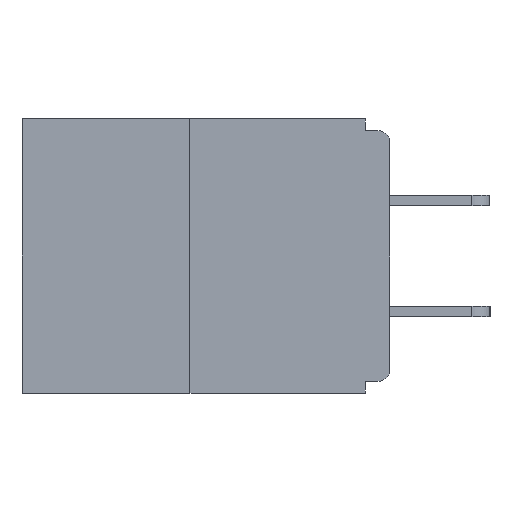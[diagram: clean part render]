
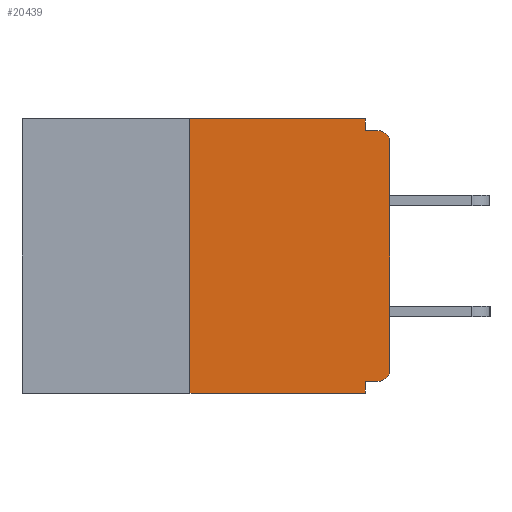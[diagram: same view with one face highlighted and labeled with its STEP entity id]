
A CAD part, left-side view. The second image highlights one B-rep face of the part: STEP entity #20439.
In plain terms, the highlighted planar face has unit normal (-1, 0, 0).
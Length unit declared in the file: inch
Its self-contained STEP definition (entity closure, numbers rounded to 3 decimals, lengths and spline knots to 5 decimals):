
#241 = CARTESIAN_POINT ( 'NONE',  ( 0., 0.015, -0.328 ) ) ;
#508 = CARTESIAN_POINT ( 'NONE',  ( 0., 0.031, -0.343 ) ) ;
#627 = LINE ( 'NONE', #2416, #22317 ) ;
#1248 = CARTESIAN_POINT ( 'NONE',  ( 0., 0., -0.03 ) ) ;
#1340 = VERTEX_POINT ( 'NONE', #13011 ) ;
#1684 = CARTESIAN_POINT ( 'NONE',  ( 0., 0.46, 0. ) ) ;
#2260 = EDGE_CURVE ( 'NONE', #18703, #17798, #22780, .T. ) ;
#2416 = CARTESIAN_POINT ( 'NONE',  ( 0., 0.031, 0. ) ) ;
#2435 = CARTESIAN_POINT ( 'NONE',  ( 0., 0.031, -0.343 ) ) ;
#2735 = VERTEX_POINT ( 'NONE', #19798 ) ;
#2969 = DIRECTION ( 'NONE',  ( -1., 0., 0. ) ) ;
#2978 = AXIS2_PLACEMENT_3D ( 'NONE', #18154, #21991, #10958 ) ;
#3700 = EDGE_CURVE ( 'NONE', #7003, #18703, #16742, .T. ) ;
#3714 = VERTEX_POINT ( 'NONE', #7396 ) ;
#3720 = DIRECTION ( 'NONE',  ( 0., 0., -1. ) ) ;
#3838 = LINE ( 'NONE', #14492, #12406 ) ;
#4538 = VECTOR ( 'NONE', #6357, 39.37008 ) ;
#4604 = EDGE_LOOP ( 'NONE', ( #6338, #17622, #10861, #5397, #20200, #6719, #4856, #18459, #21933, #16369 ) ) ;
#4856 = ORIENTED_EDGE ( 'NONE', *, *, #22133, .T. ) ;
#5397 = ORIENTED_EDGE ( 'NONE', *, *, #2260, .F. ) ;
#5763 = CARTESIAN_POINT ( 'NONE',  ( 0., 0.015, -0.015 ) ) ;
#6338 = ORIENTED_EDGE ( 'NONE', *, *, #17105, .F. ) ;
#6357 = DIRECTION ( 'NONE',  ( 0., 0., -1. ) ) ;
#6403 = AXIS2_PLACEMENT_3D ( 'NONE', #19397, #2969, #17578 ) ;
#6432 = EDGE_CURVE ( 'NONE', #20390, #17798, #19943, .T. ) ;
#6719 = ORIENTED_EDGE ( 'NONE', *, *, #13693, .T. ) ;
#6813 = DIRECTION ( 'NONE',  ( 0., 0., 1. ) ) ;
#7003 = VERTEX_POINT ( 'NONE', #241 ) ;
#7035 = CARTESIAN_POINT ( 'NONE',  ( 0., 0., -0.313 ) ) ;
#7186 = PLANE ( 'NONE',  #8529 ) ;
#7396 = CARTESIAN_POINT ( 'NONE',  ( 0., 0.031, -0.015 ) ) ;
#7540 = CIRCLE ( 'NONE', #6403, 0.015 ) ;
#8257 = VERTEX_POINT ( 'NONE', #5763 ) ;
#8529 = AXIS2_PLACEMENT_3D ( 'NONE', #1684, #16658, #3720 ) ;
#8562 = VERTEX_POINT ( 'NONE', #7035 ) ;
#8569 = DIRECTION ( 'NONE',  ( 0., -1., 0. ) ) ;
#9663 = CARTESIAN_POINT ( 'NONE',  ( 0., 0., 0. ) ) ;
#9709 = DIRECTION ( 'NONE',  ( 0., 0., -1. ) ) ;
#9779 = VECTOR ( 'NONE', #16694, 39.37008 ) ;
#10493 = LINE ( 'NONE', #16016, #18472 ) ;
#10861 = ORIENTED_EDGE ( 'NONE', *, *, #6432, .T. ) ;
#10958 = DIRECTION ( 'NONE',  ( 0., 0., -1. ) ) ;
#12406 = VECTOR ( 'NONE', #21816, 39.37008 ) ;
#13011 = CARTESIAN_POINT ( 'NONE',  ( 0., 0.25, 0. ) ) ;
#13212 = VECTOR ( 'NONE', #20590, 39.37008 ) ;
#13693 = EDGE_CURVE ( 'NONE', #7003, #8562, #7540, .T. ) ;
#14129 = EDGE_CURVE ( 'NONE', #19949, #8257, #17892, .T. ) ;
#14475 = CARTESIAN_POINT ( 'NONE',  ( 0., 0.25, 0. ) ) ;
#14489 = FACE_OUTER_BOUND ( 'NONE', #4604, .T. ) ;
#14492 = CARTESIAN_POINT ( 'NONE',  ( 0., 0., -0.015 ) ) ;
#14600 = CARTESIAN_POINT ( 'NONE',  ( 0., 0.031, -0.328 ) ) ;
#14822 = DIRECTION ( 'NONE',  ( 0., 1., 0. ) ) ;
#16016 = CARTESIAN_POINT ( 'NONE',  ( 0., 0.46, 0. ) ) ;
#16221 = CARTESIAN_POINT ( 'NONE',  ( 0., 0.46, -0.343 ) ) ;
#16369 = ORIENTED_EDGE ( 'NONE', *, *, #16873, .F. ) ;
#16658 = DIRECTION ( 'NONE',  ( 1., 0., 0. ) ) ;
#16694 = DIRECTION ( 'NONE',  ( 0., -1., 0. ) ) ;
#16742 = LINE ( 'NONE', #21331, #21065 ) ;
#16873 = EDGE_CURVE ( 'NONE', #2735, #3714, #627, .T. ) ;
#17105 = EDGE_CURVE ( 'NONE', #1340, #2735, #10493, .T. ) ;
#17578 = DIRECTION ( 'NONE',  ( 0., 0., -1. ) ) ;
#17622 = ORIENTED_EDGE ( 'NONE', *, *, #18509, .F. ) ;
#17798 = VERTEX_POINT ( 'NONE', #2435 ) ;
#17892 = CIRCLE ( 'NONE', #2978, 0.015 ) ;
#18154 = CARTESIAN_POINT ( 'NONE',  ( 0., 0.015, -0.03 ) ) ;
#18459 = ORIENTED_EDGE ( 'NONE', *, *, #14129, .T. ) ;
#18472 = VECTOR ( 'NONE', #8569, 39.37008 ) ;
#18509 = EDGE_CURVE ( 'NONE', #20390, #1340, #19886, .T. ) ;
#18551 = LINE ( 'NONE', #9663, #13212 ) ;
#18703 = VERTEX_POINT ( 'NONE', #14600 ) ;
#19397 = CARTESIAN_POINT ( 'NONE',  ( 0., 0.015, -0.313 ) ) ;
#19798 = CARTESIAN_POINT ( 'NONE',  ( 0., 0.031, 0. ) ) ;
#19886 = LINE ( 'NONE', #14475, #22663 ) ;
#19943 = LINE ( 'NONE', #16221, #9779 ) ;
#19949 = VERTEX_POINT ( 'NONE', #1248 ) ;
#20200 = ORIENTED_EDGE ( 'NONE', *, *, #3700, .F. ) ;
#20390 = VERTEX_POINT ( 'NONE', #21221 ) ;
#20439 = ADVANCED_FACE ( 'NONE', ( #14489 ), #7186, .F. ) ;
#20590 = DIRECTION ( 'NONE',  ( 0., 0., 1. ) ) ;
#21065 = VECTOR ( 'NONE', #14822, 39.37008 ) ;
#21221 = CARTESIAN_POINT ( 'NONE',  ( 0., 0.25, -0.343 ) ) ;
#21331 = CARTESIAN_POINT ( 'NONE',  ( 0., 0., -0.328 ) ) ;
#21816 = DIRECTION ( 'NONE',  ( 0., -1., 0. ) ) ;
#21933 = ORIENTED_EDGE ( 'NONE', *, *, #22804, .F. ) ;
#21991 = DIRECTION ( 'NONE',  ( -1., 0., 0. ) ) ;
#22133 = EDGE_CURVE ( 'NONE', #8562, #19949, #18551, .T. ) ;
#22317 = VECTOR ( 'NONE', #9709, 39.37008 ) ;
#22663 = VECTOR ( 'NONE', #6813, 39.37008 ) ;
#22780 = LINE ( 'NONE', #508, #4538 ) ;
#22804 = EDGE_CURVE ( 'NONE', #3714, #8257, #3838, .T. ) ;
